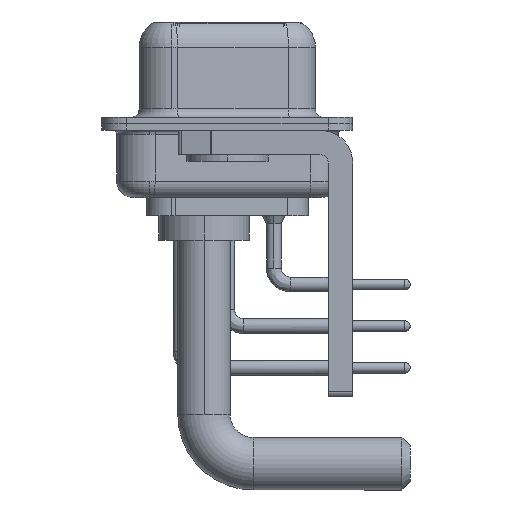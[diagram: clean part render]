
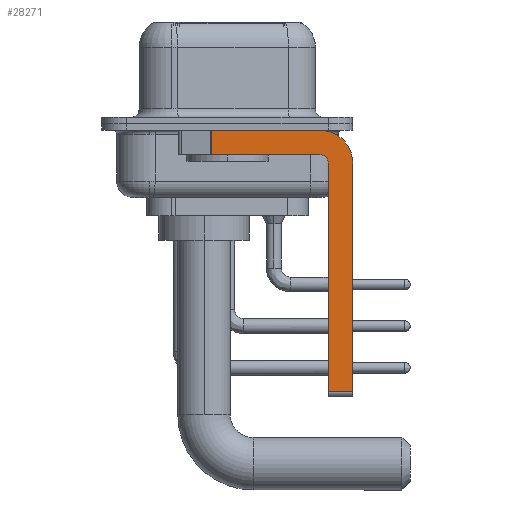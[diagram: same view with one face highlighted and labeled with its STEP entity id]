
A CAD part, left-side view. The second image highlights one B-rep face of the part: STEP entity #28271.
In plain terms, the highlighted planar face has unit normal (-1, 0, 0).
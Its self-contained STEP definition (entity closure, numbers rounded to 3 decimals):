
#284 = LINE ( 'NONE', #10654, #23750 ) ;
#501 = VERTEX_POINT ( 'NONE', #12879 ) ;
#535 = LINE ( 'NONE', #19484, #4409 ) ;
#561 = CARTESIAN_POINT ( 'NONE',  ( -2.9, -7.65, -16.35 ) ) ;
#585 = VERTEX_POINT ( 'NONE', #26901 ) ;
#1492 = LINE ( 'NONE', #22915, #15788 ) ;
#1517 = CARTESIAN_POINT ( 'NONE',  ( -2.9, -6.15, -2.4 ) ) ;
#1552 = VERTEX_POINT ( 'NONE', #28453 ) ;
#2051 = VERTEX_POINT ( 'NONE', #1517 ) ;
#2456 = VECTOR ( 'NONE', #3050, 1000. ) ;
#3050 = DIRECTION ( 'NONE',  ( 0., -1., 0. ) ) ;
#3102 = DIRECTION ( 'NONE',  ( 0., 0., -1. ) ) ;
#3401 = CARTESIAN_POINT ( 'NONE',  ( -2.9, 3., -0.4 ) ) ;
#4098 = EDGE_CURVE ( 'NONE', #1552, #13378, #1492, .T. ) ;
#4330 = ORIENTED_EDGE ( 'NONE', *, *, #20033, .F. ) ;
#4371 = CIRCLE ( 'NONE', #12788, 0.5 ) ;
#4409 = VECTOR ( 'NONE', #29708, 1000. ) ;
#4493 = ORIENTED_EDGE ( 'NONE', *, *, #7266, .F. ) ;
#4648 = EDGE_CURVE ( 'NONE', #12827, #501, #16861, .T. ) ;
#5727 = VECTOR ( 'NONE', #3102, 1000. ) ;
#6746 = CARTESIAN_POINT ( 'NONE',  ( -2.9, -5.65, -1.9 ) ) ;
#7266 = EDGE_CURVE ( 'NONE', #1552, #2051, #284, .T. ) ;
#7624 = VERTEX_POINT ( 'NONE', #34169 ) ;
#8106 = DIRECTION ( 'NONE',  ( 1., 0., 0. ) ) ;
#9802 = VECTOR ( 'NONE', #29206, 1000. ) ;
#10205 = PLANE ( 'NONE',  #16475 ) ;
#10654 = CARTESIAN_POINT ( 'NONE',  ( -2.9, -6.15, -16.6 ) ) ;
#10964 = ORIENTED_EDGE ( 'NONE', *, *, #26997, .F. ) ;
#11142 = CARTESIAN_POINT ( 'NONE',  ( -2.9, -5.65, -0.4 ) ) ;
#12788 = AXIS2_PLACEMENT_3D ( 'NONE', #28641, #34598, #21230 ) ;
#12827 = VERTEX_POINT ( 'NONE', #11142 ) ;
#12864 = DIRECTION ( 'NONE',  ( 0., 0., -1. ) ) ;
#12879 = CARTESIAN_POINT ( 'NONE',  ( -2.9, -7.65, -2.4 ) ) ;
#13232 = ORIENTED_EDGE ( 'NONE', *, *, #27360, .F. ) ;
#13378 = VERTEX_POINT ( 'NONE', #561 ) ;
#14005 = CARTESIAN_POINT ( 'NONE',  ( -2.9, -7.65, -2.4 ) ) ;
#14075 = DIRECTION ( 'NONE',  ( 0., 0., -1. ) ) ;
#15624 = EDGE_CURVE ( 'NONE', #585, #7624, #535, .T. ) ;
#15788 = VECTOR ( 'NONE', #33658, 1000. ) ;
#16475 = AXIS2_PLACEMENT_3D ( 'NONE', #20395, #33941, #12864 ) ;
#16726 = VERTEX_POINT ( 'NONE', #6746 ) ;
#16861 = CIRCLE ( 'NONE', #28666, 2. ) ;
#17137 = EDGE_LOOP ( 'NONE', ( #10964, #23425, #13232, #25399, #4493, #20430, #4330, #32600 ) ) ;
#18555 = DIRECTION ( 'NONE',  ( 0., 0., 1. ) ) ;
#19484 = CARTESIAN_POINT ( 'NONE',  ( -2.9, 0.978, -1.9 ) ) ;
#20033 = EDGE_CURVE ( 'NONE', #501, #13378, #22050, .T. ) ;
#20395 = CARTESIAN_POINT ( 'NONE',  ( -2.9, -5.65, -2.4 ) ) ;
#20430 = ORIENTED_EDGE ( 'NONE', *, *, #4098, .T. ) ;
#21230 = DIRECTION ( 'NONE',  ( 0., 0., 1. ) ) ;
#22050 = LINE ( 'NONE', #14005, #5727 ) ;
#22915 = CARTESIAN_POINT ( 'NONE',  ( -2.9, -5.65, -16.35 ) ) ;
#23425 = ORIENTED_EDGE ( 'NONE', *, *, #15624, .T. ) ;
#23750 = VECTOR ( 'NONE', #18555, 1000. ) ;
#25399 = ORIENTED_EDGE ( 'NONE', *, *, #31495, .F. ) ;
#26901 = CARTESIAN_POINT ( 'NONE',  ( -2.9, 0.978, -0.4 ) ) ;
#26997 = EDGE_CURVE ( 'NONE', #585, #12827, #30116, .T. ) ;
#27360 = EDGE_CURVE ( 'NONE', #16726, #7624, #31514, .T. ) ;
#27437 = CARTESIAN_POINT ( 'NONE',  ( -2.9, -5.65, -2.4 ) ) ;
#28271 = ADVANCED_FACE ( 'NONE', ( #34446 ), #10205, .F. ) ;
#28453 = CARTESIAN_POINT ( 'NONE',  ( -2.9, -6.15, -16.35 ) ) ;
#28641 = CARTESIAN_POINT ( 'NONE',  ( -2.9, -5.65, -2.4 ) ) ;
#28666 = AXIS2_PLACEMENT_3D ( 'NONE', #27437, #8106, #14075 ) ;
#29206 = DIRECTION ( 'NONE',  ( 0., 1., 0. ) ) ;
#29379 = CARTESIAN_POINT ( 'NONE',  ( -2.9, -5.65, -1.9 ) ) ;
#29708 = DIRECTION ( 'NONE',  ( 0., 0., -1. ) ) ;
#30116 = LINE ( 'NONE', #3401, #2456 ) ;
#31495 = EDGE_CURVE ( 'NONE', #2051, #16726, #4371, .T. ) ;
#31514 = LINE ( 'NONE', #29379, #9802 ) ;
#32600 = ORIENTED_EDGE ( 'NONE', *, *, #4648, .F. ) ;
#33658 = DIRECTION ( 'NONE',  ( 0., -1., 0. ) ) ;
#33941 = DIRECTION ( 'NONE',  ( 1., 0., 0. ) ) ;
#34169 = CARTESIAN_POINT ( 'NONE',  ( -2.9, 0.978, -1.9 ) ) ;
#34446 = FACE_OUTER_BOUND ( 'NONE', #17137, .T. ) ;
#34598 = DIRECTION ( 'NONE',  ( -1., 0., 0. ) ) ;
